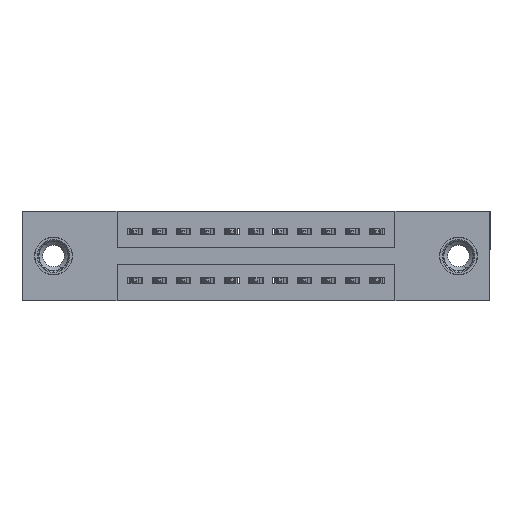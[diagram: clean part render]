
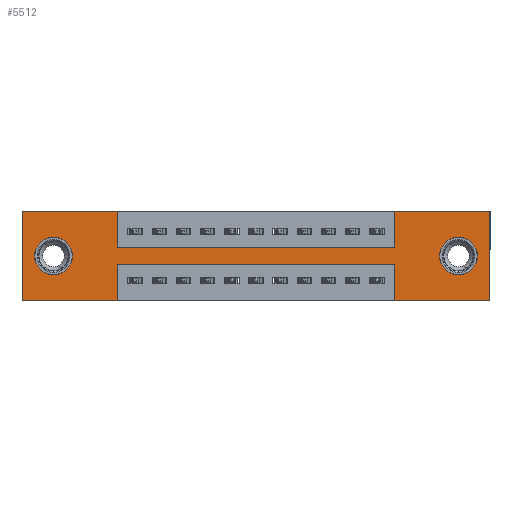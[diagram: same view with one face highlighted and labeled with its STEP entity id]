
A CAD part, front view. The second image highlights one B-rep face of the part: STEP entity #5512.
In plain terms, the highlighted planar face has unit normal (0, -1, 0).
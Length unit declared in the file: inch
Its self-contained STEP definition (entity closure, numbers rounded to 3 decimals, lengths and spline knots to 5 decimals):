
#49 = DIRECTION ( 'NONE',  ( 0., 0., -1. ) ) ;
#192 = EDGE_CURVE ( 'NONE', #14800, #4997, #9524, .T. ) ;
#222 = EDGE_CURVE ( 'NONE', #9066, #14800, #9888, .T. ) ;
#281 = DIRECTION ( 'NONE',  ( 0., 0., 1. ) ) ;
#634 = VERTEX_POINT ( 'NONE', #11645 ) ;
#732 = VERTEX_POINT ( 'NONE', #9309 ) ;
#733 = FACE_BOUND ( 'NONE', #2847, .T. ) ;
#994 = VECTOR ( 'NONE', #3604, 39.37008 ) ;
#1030 = CARTESIAN_POINT ( 'NONE',  ( 0.3925, 0., -0.15 ) ) ;
#1031 = EDGE_CURVE ( 'NONE', #8810, #12399, #14741, .T. ) ;
#1047 = VERTEX_POINT ( 'NONE', #12999 ) ;
#1204 = DIRECTION ( 'NONE',  ( -1., 0., 0. ) ) ;
#1265 = DIRECTION ( 'NONE',  ( 0., 1., 0. ) ) ;
#1483 = ORIENTED_EDGE ( 'NONE', *, *, #6255, .F. ) ;
#1576 = CARTESIAN_POINT ( 'NONE',  ( 0.3925, 0., 0. ) ) ;
#1624 = EDGE_CURVE ( 'NONE', #6438, #732, #10992, .T. ) ;
#1759 = CARTESIAN_POINT ( 'NONE',  ( 0.3925, 0., -0.22 ) ) ;
#1926 = EDGE_LOOP ( 'NONE', ( #2050, #14062 ) ) ;
#2050 = ORIENTED_EDGE ( 'NONE', *, *, #13855, .T. ) ;
#2097 = VECTOR ( 'NONE', #1204, 39.37008 ) ;
#2231 = EDGE_CURVE ( 'NONE', #7266, #13617, #9320, .T. ) ;
#2560 = PLANE ( 'NONE',  #3144 ) ;
#2827 = ORIENTED_EDGE ( 'NONE', *, *, #7238, .F. ) ;
#2847 = EDGE_LOOP ( 'NONE', ( #13967, #4679 ) ) ;
#2873 = ORIENTED_EDGE ( 'NONE', *, *, #192, .F. ) ;
#2933 = ORIENTED_EDGE ( 'NONE', *, *, #8069, .F. ) ;
#3144 = AXIS2_PLACEMENT_3D ( 'NONE', #10667, #10561, #6999 ) ;
#3181 = VECTOR ( 'NONE', #6998, 39.37008 ) ;
#3302 = CIRCLE ( 'NONE', #12996, 0.078 ) ;
#3451 = DIRECTION ( 'NONE',  ( 1., 0., 0. ) ) ;
#3604 = DIRECTION ( 'NONE',  ( 1., 0., 0. ) ) ;
#3647 = CARTESIAN_POINT ( 'NONE',  ( 1.5425, 0., -0.37 ) ) ;
#3862 = LINE ( 'NONE', #3647, #6209 ) ;
#4087 = VERTEX_POINT ( 'NONE', #7098 ) ;
#4209 = CARTESIAN_POINT ( 'NONE',  ( 0.3925, 0., -0.37 ) ) ;
#4237 = DIRECTION ( 'NONE',  ( 0., 0., -1. ) ) ;
#4288 = CARTESIAN_POINT ( 'NONE',  ( 0.3925, 0., 0. ) ) ;
#4492 = EDGE_CURVE ( 'NONE', #12018, #634, #14187, .T. ) ;
#4552 = DIRECTION ( 'NONE',  ( 0., 1., 0. ) ) ;
#4679 = ORIENTED_EDGE ( 'NONE', *, *, #1031, .T. ) ;
#4693 = CARTESIAN_POINT ( 'NONE',  ( 1.805, 0., -0.263 ) ) ;
#4837 = VERTEX_POINT ( 'NONE', #1576 ) ;
#4997 = VERTEX_POINT ( 'NONE', #6815 ) ;
#5339 = LINE ( 'NONE', #4288, #10613 ) ;
#5351 = EDGE_CURVE ( 'NONE', #1047, #4837, #13264, .T. ) ;
#5493 = LINE ( 'NONE', #7190, #10203 ) ;
#5512 = ADVANCED_FACE ( 'NONE', ( #733, #11247, #7797 ), #2560, .T. ) ;
#5576 = DIRECTION ( 'NONE',  ( -1., 0., 0. ) ) ;
#5592 = DIRECTION ( 'NONE',  ( -1., 0., 0. ) ) ;
#5731 = VECTOR ( 'NONE', #14835, 39.37008 ) ;
#5761 = VECTOR ( 'NONE', #14082, 39.37008 ) ;
#5763 = CARTESIAN_POINT ( 'NONE',  ( 0.13, 0., -0.185 ) ) ;
#6071 = VERTEX_POINT ( 'NONE', #6931 ) ;
#6209 = VECTOR ( 'NONE', #281, 39.37008 ) ;
#6252 = ORIENTED_EDGE ( 'NONE', *, *, #1624, .F. ) ;
#6255 = EDGE_CURVE ( 'NONE', #13617, #4087, #9395, .T. ) ;
#6438 = VERTEX_POINT ( 'NONE', #12358 ) ;
#6733 = DIRECTION ( 'NONE',  ( 0., 0., -1. ) ) ;
#6815 = CARTESIAN_POINT ( 'NONE',  ( 0.3925, 0., -0.37 ) ) ;
#6931 = CARTESIAN_POINT ( 'NONE',  ( 0., 0., -0.37 ) ) ;
#6998 = DIRECTION ( 'NONE',  ( 0., 0., -1. ) ) ;
#6999 = DIRECTION ( 'NONE',  ( 0., 0., -1. ) ) ;
#7098 = CARTESIAN_POINT ( 'NONE',  ( 1.5425, 0., 0. ) ) ;
#7123 = ORIENTED_EDGE ( 'NONE', *, *, #13197, .F. ) ;
#7140 = VECTOR ( 'NONE', #5592, 39.37008 ) ;
#7190 = CARTESIAN_POINT ( 'NONE',  ( 0., 0., 0. ) ) ;
#7225 = ORIENTED_EDGE ( 'NONE', *, *, #2231, .F. ) ;
#7238 = EDGE_CURVE ( 'NONE', #732, #14643, #8833, .T. ) ;
#7262 = EDGE_CURVE ( 'NONE', #6071, #1047, #9190, .T. ) ;
#7266 = VERTEX_POINT ( 'NONE', #1030 ) ;
#7280 = ORIENTED_EDGE ( 'NONE', *, *, #7262, .F. ) ;
#7721 = CARTESIAN_POINT ( 'NONE',  ( 0., 0., -0.37 ) ) ;
#7797 = FACE_OUTER_BOUND ( 'NONE', #12522, .T. ) ;
#7853 = CARTESIAN_POINT ( 'NONE',  ( 0.13, 0., -0.185 ) ) ;
#8004 = CARTESIAN_POINT ( 'NONE',  ( 0., 0., 0. ) ) ;
#8049 = VECTOR ( 'NONE', #11173, 39.37008 ) ;
#8069 = EDGE_CURVE ( 'NONE', #4087, #6438, #5493, .T. ) ;
#8404 = EDGE_CURVE ( 'NONE', #14643, #9066, #3862, .T. ) ;
#8458 = CARTESIAN_POINT ( 'NONE',  ( 0.3925, 0., -0.15 ) ) ;
#8686 = EDGE_CURVE ( 'NONE', #12399, #8810, #3302, .T. ) ;
#8810 = VERTEX_POINT ( 'NONE', #4693 ) ;
#8833 = LINE ( 'NONE', #7721, #10460 ) ;
#8880 = ORIENTED_EDGE ( 'NONE', *, *, #222, .F. ) ;
#9066 = VERTEX_POINT ( 'NONE', #13490 ) ;
#9190 = LINE ( 'NONE', #8004, #5731 ) ;
#9309 = CARTESIAN_POINT ( 'NONE',  ( 1.935, 0., -0.37 ) ) ;
#9320 = LINE ( 'NONE', #8458, #994 ) ;
#9395 = LINE ( 'NONE', #12980, #5761 ) ;
#9524 = LINE ( 'NONE', #4209, #8049 ) ;
#9752 = AXIS2_PLACEMENT_3D ( 'NONE', #7853, #12521, #12577 ) ;
#9804 = VECTOR ( 'NONE', #3451, 39.37008 ) ;
#9815 = AXIS2_PLACEMENT_3D ( 'NONE', #10658, #1265, #49 ) ;
#9835 = CARTESIAN_POINT ( 'NONE',  ( 1.805, 0., -0.107 ) ) ;
#9888 = LINE ( 'NONE', #1759, #2097 ) ;
#9930 = CARTESIAN_POINT ( 'NONE',  ( 0.3925, 0., -0.22 ) ) ;
#10203 = VECTOR ( 'NONE', #11600, 39.37008 ) ;
#10403 = CARTESIAN_POINT ( 'NONE',  ( 0., 0., 0. ) ) ;
#10450 = CARTESIAN_POINT ( 'NONE',  ( 1.935, 0., 0. ) ) ;
#10460 = VECTOR ( 'NONE', #5576, 39.37008 ) ;
#10561 = DIRECTION ( 'NONE',  ( 0., -1., 0. ) ) ;
#10613 = VECTOR ( 'NONE', #4237, 39.37008 ) ;
#10658 = CARTESIAN_POINT ( 'NONE',  ( 1.805, 0., -0.185 ) ) ;
#10667 = CARTESIAN_POINT ( 'NONE',  ( 0., 0., -0.37 ) ) ;
#10992 = LINE ( 'NONE', #10450, #3181 ) ;
#11173 = DIRECTION ( 'NONE',  ( 0., 0., -1. ) ) ;
#11247 = FACE_BOUND ( 'NONE', #1926, .T. ) ;
#11406 = CARTESIAN_POINT ( 'NONE',  ( 1.805, 0., -0.185 ) ) ;
#11600 = DIRECTION ( 'NONE',  ( 1., 0., 0. ) ) ;
#11617 = DIRECTION ( 'NONE',  ( 0., 0., 1. ) ) ;
#11643 = ORIENTED_EDGE ( 'NONE', *, *, #8404, .F. ) ;
#11645 = CARTESIAN_POINT ( 'NONE',  ( 0.13, 0., -0.107 ) ) ;
#11952 = ORIENTED_EDGE ( 'NONE', *, *, #12552, .F. ) ;
#11968 = AXIS2_PLACEMENT_3D ( 'NONE', #5763, #4552, #11617 ) ;
#12018 = VERTEX_POINT ( 'NONE', #12634 ) ;
#12358 = CARTESIAN_POINT ( 'NONE',  ( 1.935, 0., 0. ) ) ;
#12399 = VERTEX_POINT ( 'NONE', #9835 ) ;
#12521 = DIRECTION ( 'NONE',  ( 0., 1., 0. ) ) ;
#12522 = EDGE_LOOP ( 'NONE', ( #2873, #8880, #11643, #2827, #6252, #2933, #1483, #7225, #11952, #12600, #7280, #7123 ) ) ;
#12552 = EDGE_CURVE ( 'NONE', #4837, #7266, #5339, .T. ) ;
#12577 = DIRECTION ( 'NONE',  ( 0., 0., 1. ) ) ;
#12600 = ORIENTED_EDGE ( 'NONE', *, *, #5351, .F. ) ;
#12634 = CARTESIAN_POINT ( 'NONE',  ( 0.13, 0., -0.263 ) ) ;
#12740 = CIRCLE ( 'NONE', #11968, 0.078 ) ;
#12980 = CARTESIAN_POINT ( 'NONE',  ( 1.5425, 0., 0. ) ) ;
#12996 = AXIS2_PLACEMENT_3D ( 'NONE', #11406, #13884, #6733 ) ;
#12999 = CARTESIAN_POINT ( 'NONE',  ( 0., 0., 0. ) ) ;
#13197 = EDGE_CURVE ( 'NONE', #4997, #6071, #14749, .T. ) ;
#13264 = LINE ( 'NONE', #10403, #9804 ) ;
#13414 = CARTESIAN_POINT ( 'NONE',  ( 1.5425, 0., -0.15 ) ) ;
#13490 = CARTESIAN_POINT ( 'NONE',  ( 1.5425, 0., -0.22 ) ) ;
#13617 = VERTEX_POINT ( 'NONE', #13414 ) ;
#13685 = CARTESIAN_POINT ( 'NONE',  ( 0., 0., -0.37 ) ) ;
#13855 = EDGE_CURVE ( 'NONE', #634, #12018, #12740, .T. ) ;
#13884 = DIRECTION ( 'NONE',  ( 0., 1., 0. ) ) ;
#13967 = ORIENTED_EDGE ( 'NONE', *, *, #8686, .T. ) ;
#14062 = ORIENTED_EDGE ( 'NONE', *, *, #4492, .T. ) ;
#14082 = DIRECTION ( 'NONE',  ( 0., 0., 1. ) ) ;
#14187 = CIRCLE ( 'NONE', #9752, 0.078 ) ;
#14449 = CARTESIAN_POINT ( 'NONE',  ( 1.5425, 0., -0.37 ) ) ;
#14643 = VERTEX_POINT ( 'NONE', #14449 ) ;
#14741 = CIRCLE ( 'NONE', #9815, 0.078 ) ;
#14749 = LINE ( 'NONE', #13685, #7140 ) ;
#14800 = VERTEX_POINT ( 'NONE', #9930 ) ;
#14835 = DIRECTION ( 'NONE',  ( 0., 0., 1. ) ) ;
